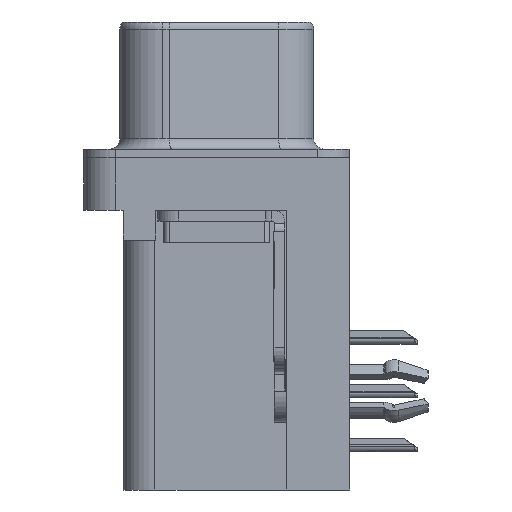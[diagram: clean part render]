
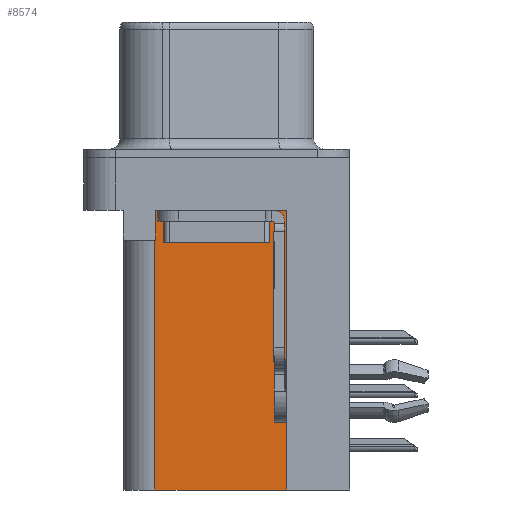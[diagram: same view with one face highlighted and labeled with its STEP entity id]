
A CAD part, left-side view. The second image highlights one B-rep face of the part: STEP entity #8574.
In plain terms, the highlighted planar face has unit normal (-1, 0, 0).
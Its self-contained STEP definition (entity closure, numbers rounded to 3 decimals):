
#284 = CARTESIAN_POINT ( 'NONE',  ( 3.79, 2.925, -3.9 ) ) ;
#623 = DIRECTION ( 'NONE',  ( 0., 1., 0. ) ) ;
#861 = VECTOR ( 'NONE', #623, 1000. ) ;
#1052 = DIRECTION ( 'NONE',  ( 0., 0., 1. ) ) ;
#3631 = LINE ( 'NONE', #6491, #861 ) ;
#4254 = VECTOR ( 'NONE', #18842, 1000. ) ;
#4446 = ORIENTED_EDGE ( 'NONE', *, *, #5793, .F. ) ;
#4812 = VECTOR ( 'NONE', #27701, 1000. ) ;
#5063 = DIRECTION ( 'NONE',  ( 0., 0., -1. ) ) ;
#5793 = EDGE_CURVE ( 'NONE', #27850, #13152, #20002, .T. ) ;
#6491 = CARTESIAN_POINT ( 'NONE',  ( 3.79, 0., -3.9 ) ) ;
#7905 = CARTESIAN_POINT ( 'NONE',  ( 3.79, 2.925, -15.7 ) ) ;
#8574 = ADVANCED_FACE ( 'NONE', ( #35339 ), #36863, .F. ) ;
#8759 = VECTOR ( 'NONE', #17225, 1000. ) ;
#9465 = EDGE_CURVE ( 'NONE', #19136, #18737, #3631, .T. ) ;
#9617 = ORIENTED_EDGE ( 'NONE', *, *, #25601, .T. ) ;
#9840 = VERTEX_POINT ( 'NONE', #30712 ) ;
#10687 = CARTESIAN_POINT ( 'NONE',  ( 3.79, -3.295, -15.7 ) ) ;
#11424 = CARTESIAN_POINT ( 'NONE',  ( 3.79, -3.295, -15.7 ) ) ;
#11791 = VECTOR ( 'NONE', #1052, 1000. ) ;
#11825 = VECTOR ( 'NONE', #5063, 1000. ) ;
#12693 = ORIENTED_EDGE ( 'NONE', *, *, #25212, .T. ) ;
#13152 = VERTEX_POINT ( 'NONE', #7905 ) ;
#14304 = DIRECTION ( 'NONE',  ( 0., 0., -1. ) ) ;
#15111 = EDGE_LOOP ( 'NONE', ( #34264, #12693, #24590, #16570, #4446, #9617 ) ) ;
#16449 = CARTESIAN_POINT ( 'NONE',  ( 3.79, 2.895, -3.9 ) ) ;
#16570 = ORIENTED_EDGE ( 'NONE', *, *, #29899, .F. ) ;
#17225 = DIRECTION ( 'NONE',  ( 0., 1., 0. ) ) ;
#18126 = EDGE_CURVE ( 'NONE', #9840, #34300, #23924, .T. ) ;
#18737 = VERTEX_POINT ( 'NONE', #284 ) ;
#18842 = DIRECTION ( 'NONE',  ( 0., 0., 1. ) ) ;
#19136 = VERTEX_POINT ( 'NONE', #36354 ) ;
#19509 = LINE ( 'NONE', #33013, #4254 ) ;
#19548 = AXIS2_PLACEMENT_3D ( 'NONE', #11424, #31254, #14304 ) ;
#20002 = LINE ( 'NONE', #10687, #4812 ) ;
#23924 = LINE ( 'NONE', #25630, #8759 ) ;
#24285 = CARTESIAN_POINT ( 'NONE',  ( 3.79, 2.895, -2.5 ) ) ;
#24590 = ORIENTED_EDGE ( 'NONE', *, *, #9465, .T. ) ;
#25149 = LINE ( 'NONE', #16449, #11825 ) ;
#25212 = EDGE_CURVE ( 'NONE', #34300, #19136, #25149, .T. ) ;
#25601 = EDGE_CURVE ( 'NONE', #27850, #9840, #26879, .T. ) ;
#25630 = CARTESIAN_POINT ( 'NONE',  ( 3.79, -3.295, -2.5 ) ) ;
#26879 = LINE ( 'NONE', #35267, #11791 ) ;
#27701 = DIRECTION ( 'NONE',  ( 0., 1., 0. ) ) ;
#27850 = VERTEX_POINT ( 'NONE', #29235 ) ;
#29235 = CARTESIAN_POINT ( 'NONE',  ( 3.79, -3.295, -15.7 ) ) ;
#29899 = EDGE_CURVE ( 'NONE', #13152, #18737, #19509, .T. ) ;
#30712 = CARTESIAN_POINT ( 'NONE',  ( 3.79, -3.295, -2.5 ) ) ;
#31254 = DIRECTION ( 'NONE',  ( 1., 0., 0. ) ) ;
#33013 = CARTESIAN_POINT ( 'NONE',  ( 3.79, 2.925, -15.7 ) ) ;
#34264 = ORIENTED_EDGE ( 'NONE', *, *, #18126, .T. ) ;
#34300 = VERTEX_POINT ( 'NONE', #24285 ) ;
#35267 = CARTESIAN_POINT ( 'NONE',  ( 3.79, -3.295, -15.7 ) ) ;
#35339 = FACE_OUTER_BOUND ( 'NONE', #15111, .T. ) ;
#36354 = CARTESIAN_POINT ( 'NONE',  ( 3.79, 2.895, -3.9 ) ) ;
#36863 = PLANE ( 'NONE',  #19548 ) ;
